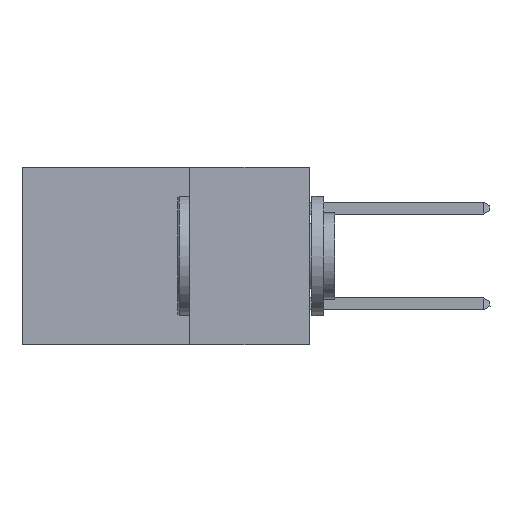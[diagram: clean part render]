
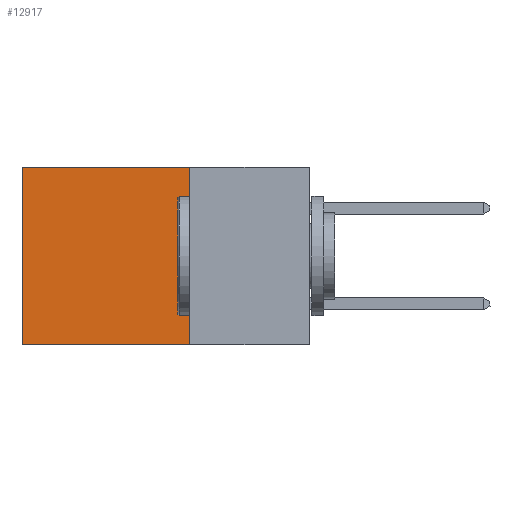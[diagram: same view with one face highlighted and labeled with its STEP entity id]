
A CAD part, left-side view. The second image highlights one B-rep face of the part: STEP entity #12917.
In plain terms, the highlighted planar face has unit normal (-1, 0, 0).
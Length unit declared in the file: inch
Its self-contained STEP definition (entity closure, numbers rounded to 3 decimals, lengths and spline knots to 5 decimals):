
#788 = DIRECTION ( 'NONE',  ( 1., 0., 0. ) ) ;
#804 = VECTOR ( 'NONE', #3731, 39.37008 ) ;
#1294 = LINE ( 'NONE', #3660, #5192 ) ;
#1344 = EDGE_CURVE ( 'NONE', #8476, #3437, #18345, .T. ) ;
#1345 = EDGE_CURVE ( 'NONE', #15312, #3437, #1294, .T. ) ;
#2720 = EDGE_LOOP ( 'NONE', ( #4135, #7403, #16827, #6626 ) ) ;
#2798 = VECTOR ( 'NONE', #21093, 39.37008 ) ;
#2869 = VERTEX_POINT ( 'NONE', #4465 ) ;
#3273 = CARTESIAN_POINT ( 'NONE',  ( 0.2875, 0.25, -0.37 ) ) ;
#3336 = LINE ( 'NONE', #14582, #2798 ) ;
#3437 = VERTEX_POINT ( 'NONE', #7108 ) ;
#3660 = CARTESIAN_POINT ( 'NONE',  ( 0.2875, 0.25, -0.37 ) ) ;
#3731 = DIRECTION ( 'NONE',  ( 0., 0., -1. ) ) ;
#3965 = DIRECTION ( 'NONE',  ( 0., 1., 0. ) ) ;
#3999 = LINE ( 'NONE', #5741, #11780 ) ;
#4116 = CARTESIAN_POINT ( 'NONE',  ( 0.2875, 0.6, 0. ) ) ;
#4135 = ORIENTED_EDGE ( 'NONE', *, *, #1344, .T. ) ;
#4465 = CARTESIAN_POINT ( 'NONE',  ( 0.2875, 0.25, 0. ) ) ;
#5192 = VECTOR ( 'NONE', #3965, 39.37008 ) ;
#5702 = CARTESIAN_POINT ( 'NONE',  ( 0.2875, 0.25, 0. ) ) ;
#5741 = CARTESIAN_POINT ( 'NONE',  ( 0.2875, 0.25, 0. ) ) ;
#6626 = ORIENTED_EDGE ( 'NONE', *, *, #19990, .T. ) ;
#7108 = CARTESIAN_POINT ( 'NONE',  ( 0.2875, 0.6, -0.37 ) ) ;
#7403 = ORIENTED_EDGE ( 'NONE', *, *, #1345, .F. ) ;
#8476 = VERTEX_POINT ( 'NONE', #18827 ) ;
#10746 = PLANE ( 'NONE',  #14326 ) ;
#11780 = VECTOR ( 'NONE', #20544, 39.37008 ) ;
#12379 = DIRECTION ( 'NONE',  ( 0., 0., -1. ) ) ;
#12917 = ADVANCED_FACE ( 'NONE', ( #13957 ), #10746, .F. ) ;
#13715 = EDGE_CURVE ( 'NONE', #2869, #15312, #3336, .T. ) ;
#13957 = FACE_OUTER_BOUND ( 'NONE', #2720, .T. ) ;
#14326 = AXIS2_PLACEMENT_3D ( 'NONE', #5702, #788, #12379 ) ;
#14582 = CARTESIAN_POINT ( 'NONE',  ( 0.2875, 0.25, 0. ) ) ;
#15312 = VERTEX_POINT ( 'NONE', #3273 ) ;
#16827 = ORIENTED_EDGE ( 'NONE', *, *, #13715, .F. ) ;
#18345 = LINE ( 'NONE', #4116, #804 ) ;
#18827 = CARTESIAN_POINT ( 'NONE',  ( 0.2875, 0.6, 0. ) ) ;
#19990 = EDGE_CURVE ( 'NONE', #2869, #8476, #3999, .T. ) ;
#20544 = DIRECTION ( 'NONE',  ( 0., 1., 0. ) ) ;
#21093 = DIRECTION ( 'NONE',  ( 0., 0., -1. ) ) ;
